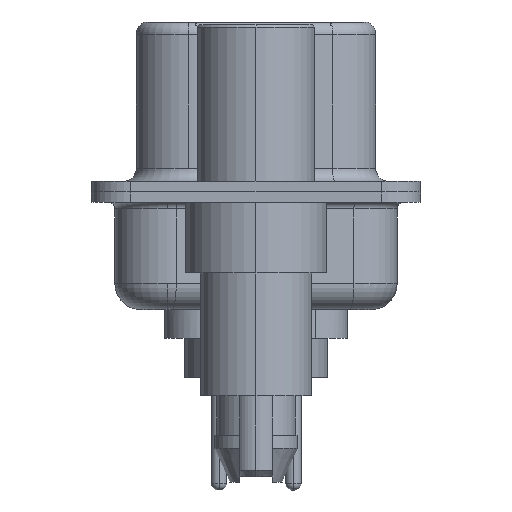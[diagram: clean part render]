
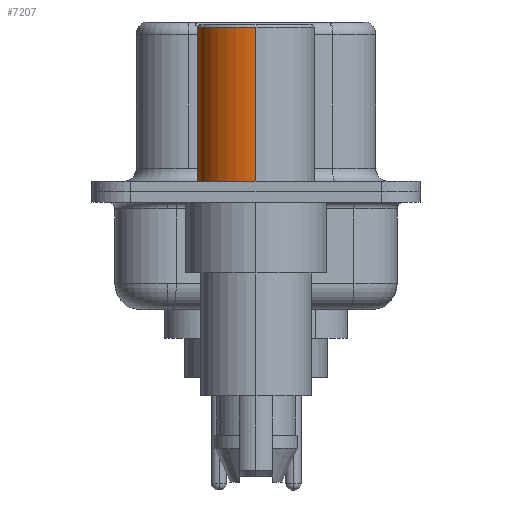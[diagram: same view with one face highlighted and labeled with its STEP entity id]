
A CAD part, left-side view. The second image highlights one B-rep face of the part: STEP entity #7207.
In plain terms, the highlighted cylindrical face has radius 2.25 mm (diameter 4.5 mm), a partial arc.
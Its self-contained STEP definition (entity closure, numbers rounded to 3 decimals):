
#1119 = CARTESIAN_POINT ( 'NONE',  ( 0., 0., 0.4 ) ) ;
#2015 = DIRECTION ( 'NONE',  ( 0., 0., 1. ) ) ;
#2100 = VECTOR ( 'NONE', #3902, 1000. ) ;
#3061 = DIRECTION ( 'NONE',  ( 1., 0., 0. ) ) ;
#3077 = VERTEX_POINT ( 'NONE', #17654 ) ;
#3322 = CARTESIAN_POINT ( 'NONE',  ( 0., 0., 6.3 ) ) ;
#3527 = ORIENTED_EDGE ( 'NONE', *, *, #22224, .F. ) ;
#3902 = DIRECTION ( 'NONE',  ( 0., 0., 1. ) ) ;
#4509 = VECTOR ( 'NONE', #10025, 1000. ) ;
#4640 = EDGE_LOOP ( 'NONE', ( #12965, #5882, #3527, #7624 ) ) ;
#4869 = CARTESIAN_POINT ( 'NONE',  ( -2.25, 0., 6.3 ) ) ;
#5134 = CIRCLE ( 'NONE', #10307, 2.25 ) ;
#5267 = DIRECTION ( 'NONE',  ( 1., 0., 0. ) ) ;
#5532 = AXIS2_PLACEMENT_3D ( 'NONE', #19319, #2015, #7704 ) ;
#5882 = ORIENTED_EDGE ( 'NONE', *, *, #12151, .T. ) ;
#7207 = ADVANCED_FACE ( 'NONE', ( #14470 ), #24155, .T. ) ;
#7492 = EDGE_CURVE ( 'NONE', #14373, #3077, #9615, .T. ) ;
#7624 = ORIENTED_EDGE ( 'NONE', *, *, #7492, .F. ) ;
#7704 = DIRECTION ( 'NONE',  ( 1., 0., 0. ) ) ;
#9615 = LINE ( 'NONE', #19643, #4509 ) ;
#9806 = CARTESIAN_POINT ( 'NONE',  ( -2.25, 0., 0.581 ) ) ;
#10025 = DIRECTION ( 'NONE',  ( 0., 0., 1. ) ) ;
#10307 = AXIS2_PLACEMENT_3D ( 'NONE', #1119, #14636, #3061 ) ;
#12151 = EDGE_CURVE ( 'NONE', #19145, #24828, #22077, .T. ) ;
#12965 = ORIENTED_EDGE ( 'NONE', *, *, #20270, .T. ) ;
#14373 = VERTEX_POINT ( 'NONE', #17194 ) ;
#14470 = FACE_OUTER_BOUND ( 'NONE', #4640, .T. ) ;
#14636 = DIRECTION ( 'NONE',  ( 0., 0., 1. ) ) ;
#15007 = CIRCLE ( 'NONE', #22479, 2.25 ) ;
#16827 = DIRECTION ( 'NONE',  ( 0., 0., 1. ) ) ;
#17194 = CARTESIAN_POINT ( 'NONE',  ( 2.25, 0., 0.4 ) ) ;
#17654 = CARTESIAN_POINT ( 'NONE',  ( 2.25, 0., 6.3 ) ) ;
#19145 = VERTEX_POINT ( 'NONE', #20367 ) ;
#19319 = CARTESIAN_POINT ( 'NONE',  ( 0., 0., 0.581 ) ) ;
#19643 = CARTESIAN_POINT ( 'NONE',  ( 2.25, 0., 0.581 ) ) ;
#20270 = EDGE_CURVE ( 'NONE', #14373, #19145, #5134, .T. ) ;
#20367 = CARTESIAN_POINT ( 'NONE',  ( -2.25, 0., 0.4 ) ) ;
#22077 = LINE ( 'NONE', #9806, #2100 ) ;
#22224 = EDGE_CURVE ( 'NONE', #3077, #24828, #15007, .T. ) ;
#22479 = AXIS2_PLACEMENT_3D ( 'NONE', #3322, #16827, #5267 ) ;
#24155 = CYLINDRICAL_SURFACE ( 'NONE', #5532, 2.25 ) ;
#24828 = VERTEX_POINT ( 'NONE', #4869 ) ;
